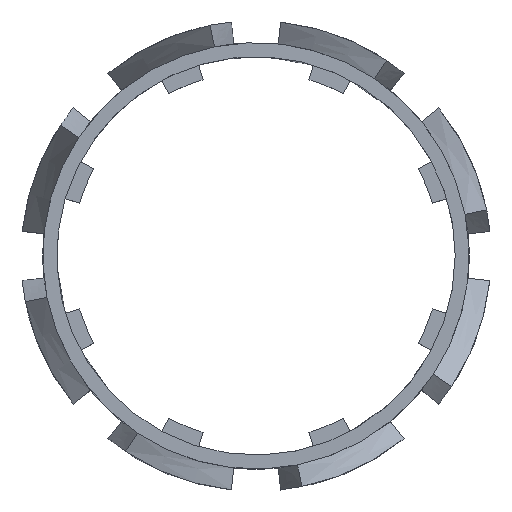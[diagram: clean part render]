
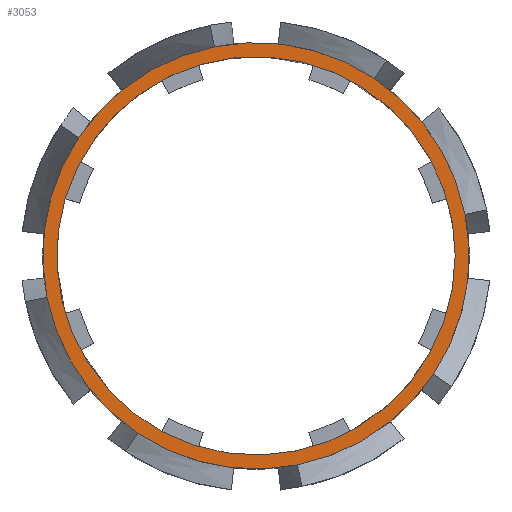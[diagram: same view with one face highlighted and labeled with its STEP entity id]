
A CAD part, top view. The second image highlights one B-rep face of the part: STEP entity #3053.
In plain terms, the highlighted planar face has unit normal (0, 0, 1).
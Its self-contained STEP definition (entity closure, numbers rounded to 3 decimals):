
#113=CARTESIAN_POINT('',(27.1,0.,20.0));
#114=VERTEX_POINT('',#113);
#115=CARTESIAN_POINT('',(0.0,0.0,20.0));
#116=DIRECTION('',(0.0,0.0,-1.0));
#117=DIRECTION('',(-1.0,0.0,0.0));
#118=AXIS2_PLACEMENT_3D('',#115,#116,#117);
#119=CIRCLE('',#118,27.1);
#120=EDGE_CURVE('',#114,#114,#119,.T.);
#1485=CARTESIAN_POINT('',(-16.112,-24.113,20.));
#1486=VERTEX_POINT('',#1485);
#1540=CARTESIAN_POINT('',(-28.443,-5.658,20.));
#1541=VERTEX_POINT('',#1540);
#1641=CARTESIAN_POINT('',(-24.113,16.112,20.));
#1642=VERTEX_POINT('',#1641);
#1742=CARTESIAN_POINT('',(-5.658,28.443,20.));
#1743=VERTEX_POINT('',#1742);
#1843=CARTESIAN_POINT('',(16.112,24.113,20.));
#1844=VERTEX_POINT('',#1843);
#1944=CARTESIAN_POINT('',(28.443,5.658,20.));
#1945=VERTEX_POINT('',#1944);
#2045=CARTESIAN_POINT('',(24.113,-16.112,20.));
#2046=VERTEX_POINT('',#2045);
#2146=CARTESIAN_POINT('',(5.658,-28.443,20.));
#2147=VERTEX_POINT('',#2146);
#2243=CARTESIAN_POINT('',(0.0,0.0,20.0));
#2244=DIRECTION('',(0.0,0.0,1.0));
#2245=DIRECTION('',(0.707,-0.707,0.0));
#2246=AXIS2_PLACEMENT_3D('',#2243,#2244,#2245);
#2247=CIRCLE('',#2246,29.0);
#2248=EDGE_CURVE('',#1541,#1486,#2247,.T.);
#2344=CARTESIAN_POINT('',(0.0,0.0,20.0));
#2345=DIRECTION('',(0.0,0.0,1.0));
#2346=DIRECTION('',(0.0,-1.0,0.0));
#2347=AXIS2_PLACEMENT_3D('',#2344,#2345,#2346);
#2348=CIRCLE('',#2347,29.);
#2349=EDGE_CURVE('',#1642,#1541,#2348,.T.);
#2445=CARTESIAN_POINT('',(0.0,0.0,20.0));
#2446=DIRECTION('',(0.0,0.0,1.0));
#2447=DIRECTION('',(-0.707,-0.707,0.0));
#2448=AXIS2_PLACEMENT_3D('',#2445,#2446,#2447);
#2449=CIRCLE('',#2448,29.0);
#2450=EDGE_CURVE('',#1743,#1642,#2449,.T.);
#2546=CARTESIAN_POINT('',(0.0,0.0,20.0));
#2547=DIRECTION('',(0.0,0.0,1.0));
#2548=DIRECTION('',(-1.0,0.0,0.0));
#2549=AXIS2_PLACEMENT_3D('',#2546,#2547,#2548);
#2550=CIRCLE('',#2549,29.);
#2551=EDGE_CURVE('',#1844,#1743,#2550,.T.);
#2647=CARTESIAN_POINT('',(0.0,0.0,20.0));
#2648=DIRECTION('',(0.0,0.0,1.0));
#2649=DIRECTION('',(-0.707,0.707,0.0));
#2650=AXIS2_PLACEMENT_3D('',#2647,#2648,#2649);
#2651=CIRCLE('',#2650,29.);
#2652=EDGE_CURVE('',#1945,#1844,#2651,.T.);
#2748=CARTESIAN_POINT('',(0.0,0.0,20.0));
#2749=DIRECTION('',(0.0,0.0,1.0));
#2750=DIRECTION('',(0.0,1.0,0.0));
#2751=AXIS2_PLACEMENT_3D('',#2748,#2749,#2750);
#2752=CIRCLE('',#2751,29.);
#2753=EDGE_CURVE('',#2046,#1945,#2752,.T.);
#2849=CARTESIAN_POINT('',(0.0,0.0,20.0));
#2850=DIRECTION('',(0.0,0.0,1.0));
#2851=DIRECTION('',(0.707,0.707,0.0));
#2852=AXIS2_PLACEMENT_3D('',#2849,#2850,#2851);
#2853=CIRCLE('',#2852,29.);
#2854=EDGE_CURVE('',#2147,#2046,#2853,.T.);
#2977=CARTESIAN_POINT('',(0.0,0.0,20.0));
#2978=DIRECTION('',(0.0,0.0,1.0));
#2979=DIRECTION('',(1.0,0.0,0.0));
#2980=AXIS2_PLACEMENT_3D('',#2977,#2978,#2979);
#2981=CIRCLE('',#2980,29.);
#2982=EDGE_CURVE('',#1486,#2147,#2981,.T.);
#3035=CARTESIAN_POINT('',(0.0,0.0,20.0));
#3036=DIRECTION('',(0.0,0.0,-1.0));
#3037=DIRECTION('',(-1.0,0.0,0.0));
#3038=AXIS2_PLACEMENT_3D('',#3035,#3036,#3037);
#3039=PLANE('',#3038);
#3040=ORIENTED_EDGE('',*,*,#2248,.T.);
#3041=ORIENTED_EDGE('',*,*,#2982,.T.);
#3042=ORIENTED_EDGE('',*,*,#2854,.T.);
#3043=ORIENTED_EDGE('',*,*,#2753,.T.);
#3044=ORIENTED_EDGE('',*,*,#2652,.T.);
#3045=ORIENTED_EDGE('',*,*,#2551,.T.);
#3046=ORIENTED_EDGE('',*,*,#2450,.T.);
#3047=ORIENTED_EDGE('',*,*,#2349,.T.);
#3048=EDGE_LOOP('',(#3040,#3041,#3042,#3043,#3044,#3045,#3046,#3047));
#3049=FACE_OUTER_BOUND('',#3048,.T.);
#3050=ORIENTED_EDGE('',*,*,#120,.T.);
#3051=EDGE_LOOP('',(#3050));
#3052=FACE_BOUND('',#3051,.T.);
#3053=ADVANCED_FACE('',(#3049,#3052),#3039,.F.);
